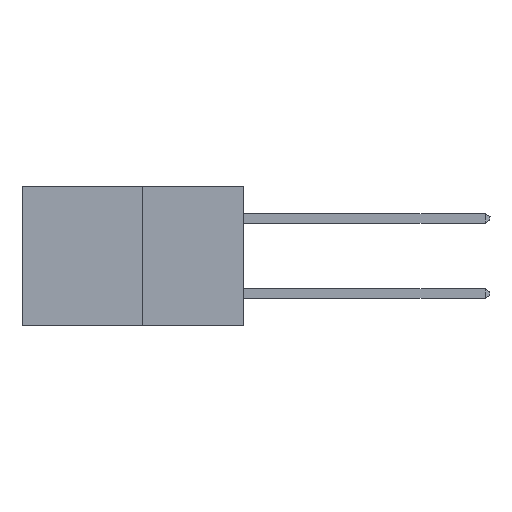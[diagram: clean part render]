
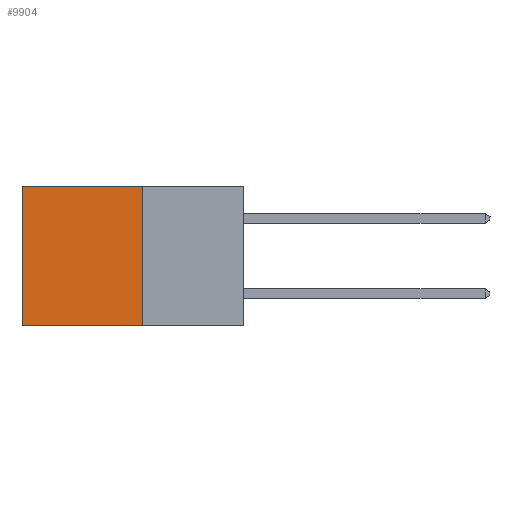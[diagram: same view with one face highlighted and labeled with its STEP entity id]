
A CAD part, left-side view. The second image highlights one B-rep face of the part: STEP entity #9904.
In plain terms, the highlighted planar face has unit normal (-1, 0, 0).
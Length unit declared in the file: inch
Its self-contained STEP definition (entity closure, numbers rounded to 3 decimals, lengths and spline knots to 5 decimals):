
#206 = CARTESIAN_POINT ( 'NONE',  ( 0.277, 0.27, -0.37 ) ) ;
#766 = CARTESIAN_POINT ( 'NONE',  ( 0.277, 0.27, -0.37 ) ) ;
#2174 = DIRECTION ( 'NONE',  ( 0., 0., -1. ) ) ;
#2592 = CARTESIAN_POINT ( 'NONE',  ( 0.277, 0.59, 0. ) ) ;
#2765 = DIRECTION ( 'NONE',  ( 0., 0., -1. ) ) ;
#3598 = EDGE_CURVE ( 'NONE', #6299, #9272, #11246, .T. ) ;
#3721 = LINE ( 'NONE', #766, #10855 ) ;
#4055 = EDGE_CURVE ( 'NONE', #8959, #16726, #10812, .T. ) ;
#4334 = ORIENTED_EDGE ( 'NONE', *, *, #3598, .T. ) ;
#4809 = DIRECTION ( 'NONE',  ( 0., 1., 0. ) ) ;
#5062 = CARTESIAN_POINT ( 'NONE',  ( 0.277, 0.27, -0.37 ) ) ;
#5071 = VECTOR ( 'NONE', #10068, 39.37008 ) ;
#6036 = CARTESIAN_POINT ( 'NONE',  ( 0.277, 0.59, -0.37 ) ) ;
#6118 = CARTESIAN_POINT ( 'NONE',  ( 0.277, 0.27, 0. ) ) ;
#6299 = VERTEX_POINT ( 'NONE', #15482 ) ;
#6777 = CARTESIAN_POINT ( 'NONE',  ( 0.277, 0.27, -0.37 ) ) ;
#8959 = VERTEX_POINT ( 'NONE', #5062 ) ;
#9092 = CARTESIAN_POINT ( 'NONE',  ( 0.277, 0.59, -0.37 ) ) ;
#9272 = VERTEX_POINT ( 'NONE', #2592 ) ;
#9305 = EDGE_LOOP ( 'NONE', ( #14733, #9777, #11034, #4334 ) ) ;
#9777 = ORIENTED_EDGE ( 'NONE', *, *, #4055, .F. ) ;
#9904 = ADVANCED_FACE ( 'NONE', ( #14278 ), #10743, .F. ) ;
#10068 = DIRECTION ( 'NONE',  ( 0., 0., -1. ) ) ;
#10743 = PLANE ( 'NONE',  #13352 ) ;
#10796 = DIRECTION ( 'NONE',  ( 1., 0., 0. ) ) ;
#10812 = LINE ( 'NONE', #206, #14727 ) ;
#10855 = VECTOR ( 'NONE', #2174, 39.37008 ) ;
#10925 = EDGE_CURVE ( 'NONE', #9272, #16726, #16073, .T. ) ;
#11034 = ORIENTED_EDGE ( 'NONE', *, *, #13913, .F. ) ;
#11053 = DIRECTION ( 'NONE',  ( 0., 1., 0. ) ) ;
#11246 = LINE ( 'NONE', #6118, #14334 ) ;
#13352 = AXIS2_PLACEMENT_3D ( 'NONE', #6777, #10796, #2765 ) ;
#13913 = EDGE_CURVE ( 'NONE', #6299, #8959, #3721, .T. ) ;
#14278 = FACE_OUTER_BOUND ( 'NONE', #9305, .T. ) ;
#14334 = VECTOR ( 'NONE', #4809, 39.37008 ) ;
#14727 = VECTOR ( 'NONE', #11053, 39.37008 ) ;
#14733 = ORIENTED_EDGE ( 'NONE', *, *, #10925, .T. ) ;
#15482 = CARTESIAN_POINT ( 'NONE',  ( 0.277, 0.27, 0. ) ) ;
#16073 = LINE ( 'NONE', #6036, #5071 ) ;
#16726 = VERTEX_POINT ( 'NONE', #9092 ) ;
